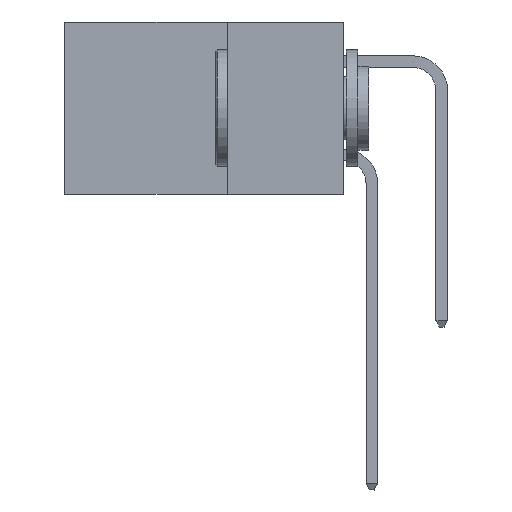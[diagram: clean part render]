
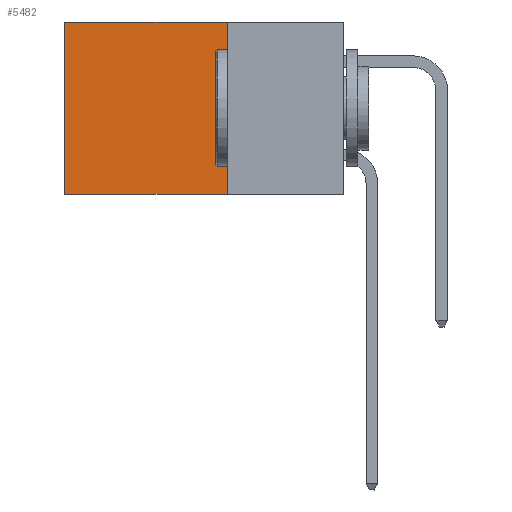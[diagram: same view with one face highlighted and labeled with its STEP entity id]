
A CAD part, left-side view. The second image highlights one B-rep face of the part: STEP entity #5482.
In plain terms, the highlighted planar face has unit normal (-1, 0, 0).
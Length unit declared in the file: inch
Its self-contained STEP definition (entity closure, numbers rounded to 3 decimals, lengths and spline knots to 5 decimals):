
#2616 = EDGE_CURVE ( 'NONE', #12637, #6559, #13048, .T. ) ;
#3738 = LINE ( 'NONE', #12582, #14161 ) ;
#3793 = CARTESIAN_POINT ( 'NONE',  ( 0.298, 0.6, -0.37 ) ) ;
#3972 = VECTOR ( 'NONE', #17589, 39.37008 ) ;
#4269 = CARTESIAN_POINT ( 'NONE',  ( 0.298, 0.25, 0. ) ) ;
#4385 = DIRECTION ( 'NONE',  ( 0., 0., -1. ) ) ;
#4388 = PLANE ( 'NONE',  #11778 ) ;
#4460 = DIRECTION ( 'NONE',  ( 0., 1., 0. ) ) ;
#4777 = DIRECTION ( 'NONE',  ( 0., 1., 0. ) ) ;
#5299 = EDGE_CURVE ( 'NONE', #6559, #14265, #16933, .T. ) ;
#5482 = ADVANCED_FACE ( 'NONE', ( #12648 ), #4388, .F. ) ;
#5505 = VECTOR ( 'NONE', #4385, 39.37008 ) ;
#5938 = LINE ( 'NONE', #12507, #5505 ) ;
#6559 = VERTEX_POINT ( 'NONE', #16913 ) ;
#6996 = DIRECTION ( 'NONE',  ( 1., 0., 0. ) ) ;
#7230 = DIRECTION ( 'NONE',  ( 0., 0., -1. ) ) ;
#8319 = ORIENTED_EDGE ( 'NONE', *, *, #10409, .F. ) ;
#9069 = EDGE_CURVE ( 'NONE', #12637, #13622, #5938, .T. ) ;
#9457 = VECTOR ( 'NONE', #4777, 39.37008 ) ;
#10084 = ORIENTED_EDGE ( 'NONE', *, *, #9069, .F. ) ;
#10409 = EDGE_CURVE ( 'NONE', #13622, #14265, #3738, .T. ) ;
#10866 = ORIENTED_EDGE ( 'NONE', *, *, #5299, .T. ) ;
#11778 = AXIS2_PLACEMENT_3D ( 'NONE', #4269, #6996, #7230 ) ;
#11816 = ORIENTED_EDGE ( 'NONE', *, *, #2616, .T. ) ;
#12271 = CARTESIAN_POINT ( 'NONE',  ( 0.298, 0.6, 0. ) ) ;
#12507 = CARTESIAN_POINT ( 'NONE',  ( 0.298, 0.25, 0. ) ) ;
#12582 = CARTESIAN_POINT ( 'NONE',  ( 0.298, 0.25, -0.37 ) ) ;
#12609 = CARTESIAN_POINT ( 'NONE',  ( 0.298, 0.25, 0. ) ) ;
#12637 = VERTEX_POINT ( 'NONE', #12609 ) ;
#12648 = FACE_OUTER_BOUND ( 'NONE', #12929, .T. ) ;
#12929 = EDGE_LOOP ( 'NONE', ( #10866, #8319, #10084, #11816 ) ) ;
#13048 = LINE ( 'NONE', #14330, #9457 ) ;
#13622 = VERTEX_POINT ( 'NONE', #15833 ) ;
#14161 = VECTOR ( 'NONE', #4460, 39.37008 ) ;
#14265 = VERTEX_POINT ( 'NONE', #3793 ) ;
#14330 = CARTESIAN_POINT ( 'NONE',  ( 0.298, 0.25, 0. ) ) ;
#15833 = CARTESIAN_POINT ( 'NONE',  ( 0.298, 0.25, -0.37 ) ) ;
#16913 = CARTESIAN_POINT ( 'NONE',  ( 0.298, 0.6, 0. ) ) ;
#16933 = LINE ( 'NONE', #12271, #3972 ) ;
#17589 = DIRECTION ( 'NONE',  ( 0., 0., -1. ) ) ;
